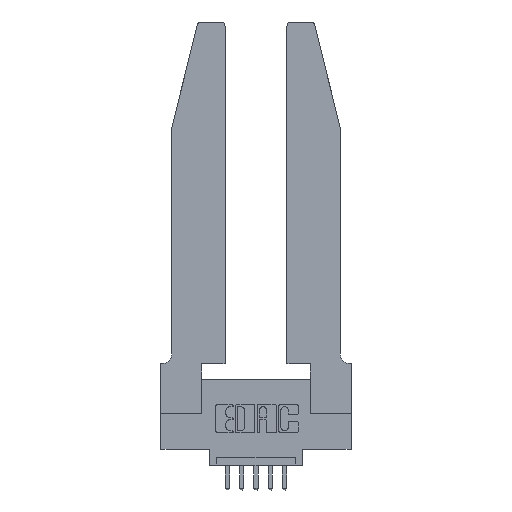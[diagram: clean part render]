
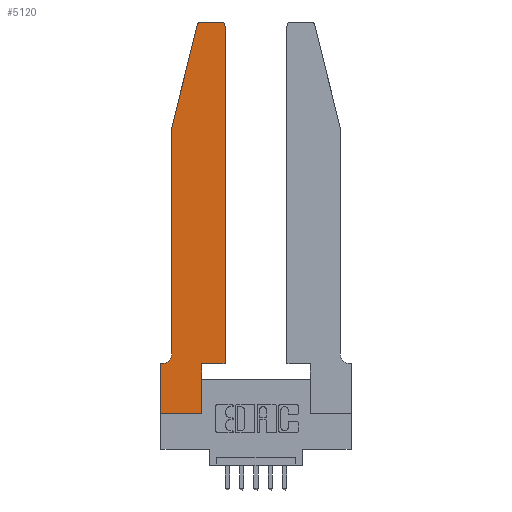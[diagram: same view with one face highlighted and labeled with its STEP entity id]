
A CAD part, top view. The second image highlights one B-rep face of the part: STEP entity #5120.
In plain terms, the highlighted planar face has unit normal (0, 0, 1).
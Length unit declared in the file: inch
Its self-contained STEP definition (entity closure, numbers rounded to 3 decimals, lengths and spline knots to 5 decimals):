
#162 = CARTESIAN_POINT ( 'NONE',  ( 0.2865, 0.35, 0.37 ) ) ;
#192 = EDGE_LOOP ( 'NONE', ( #10039, #7014, #6749, #9158, #2824, #9140, #12492, #2630, #3461, #7036, #6028, #13361 ) ) ;
#282 = CARTESIAN_POINT ( 'NONE',  ( 0., 0.35, 0.37 ) ) ;
#284 = DIRECTION ( 'NONE',  ( -0.239, -0.971, 0. ) ) ;
#394 = VERTEX_POINT ( 'NONE', #13601 ) ;
#401 = LINE ( 'NONE', #1565, #3555 ) ;
#539 = VECTOR ( 'NONE', #2109, 39.37008 ) ;
#833 = VERTEX_POINT ( 'NONE', #4978 ) ;
#885 = DIRECTION ( 'NONE',  ( 0., 0., 1. ) ) ;
#1018 = VECTOR ( 'NONE', #3364, 39.37008 ) ;
#1090 = AXIS2_PLACEMENT_3D ( 'NONE', #282, #4609, #3397 ) ;
#1137 = VERTEX_POINT ( 'NONE', #2534 ) ;
#1203 = VERTEX_POINT ( 'NONE', #13426 ) ;
#1565 = CARTESIAN_POINT ( 'NONE',  ( 0.0755, 0.35, 0.37 ) ) ;
#1767 = VECTOR ( 'NONE', #12735, 39.37008 ) ;
#1770 = VECTOR ( 'NONE', #7680, 39.37008 ) ;
#1950 = AXIS2_PLACEMENT_3D ( 'NONE', #2578, #2714, #5833 ) ;
#2034 = DIRECTION ( 'NONE',  ( 1., 0., 0. ) ) ;
#2109 = DIRECTION ( 'NONE',  ( 0., -1., 0. ) ) ;
#2235 = CARTESIAN_POINT ( 'NONE',  ( 0.2605, 2.75, 0.37 ) ) ;
#2374 = DIRECTION ( 'NONE',  ( -1., 0., 0. ) ) ;
#2534 = CARTESIAN_POINT ( 'NONE',  ( 0.2865, 0.35, 0.37 ) ) ;
#2578 = CARTESIAN_POINT ( 'NONE',  ( 0.4205, 2.72, 0.37 ) ) ;
#2630 = ORIENTED_EDGE ( 'NONE', *, *, #3202, .T. ) ;
#2714 = DIRECTION ( 'NONE',  ( 0., 0., 1. ) ) ;
#2824 = ORIENTED_EDGE ( 'NONE', *, *, #10400, .T. ) ;
#2969 = CARTESIAN_POINT ( 'NONE',  ( 0., 0., 0.37 ) ) ;
#3109 = CARTESIAN_POINT ( 'NONE',  ( 0.284, 2.72, 0.37 ) ) ;
#3128 = LINE ( 'NONE', #13609, #9142 ) ;
#3202 = EDGE_CURVE ( 'NONE', #12722, #394, #4617, .T. ) ;
#3364 = DIRECTION ( 'NONE',  ( 0., 1., 0. ) ) ;
#3397 = DIRECTION ( 'NONE',  ( 1., 0., 0. ) ) ;
#3461 = ORIENTED_EDGE ( 'NONE', *, *, #12194, .T. ) ;
#3555 = VECTOR ( 'NONE', #13127, 39.37008 ) ;
#3591 = VERTEX_POINT ( 'NONE', #9703 ) ;
#3933 = LINE ( 'NONE', #9769, #1770 ) ;
#4102 = DIRECTION ( 'NONE',  ( 1., 0., 0. ) ) ;
#4292 = DIRECTION ( 'NONE',  ( 0., 0., -1. ) ) ;
#4609 = DIRECTION ( 'NONE',  ( 0., 0., 1. ) ) ;
#4617 = LINE ( 'NONE', #2969, #1767 ) ;
#4635 = CARTESIAN_POINT ( 'NONE',  ( 0.0055, 0.35, 0.37 ) ) ;
#4761 = CARTESIAN_POINT ( 'NONE',  ( 0.4205, 2.75, 0.37 ) ) ;
#4847 = VECTOR ( 'NONE', #7416, 39.37008 ) ;
#4978 = CARTESIAN_POINT ( 'NONE',  ( 0.4505, 2.72, 0.37 ) ) ;
#5034 = CARTESIAN_POINT ( 'NONE',  ( 0.284, 2.75, 0.37 ) ) ;
#5111 = CARTESIAN_POINT ( 'NONE',  ( 0., 0., 0.37 ) ) ;
#5120 = ADVANCED_FACE ( 'NONE', ( #7753 ), #7647, .T. ) ;
#5221 = EDGE_CURVE ( 'NONE', #11768, #3591, #401, .T. ) ;
#5291 = CARTESIAN_POINT ( 'NONE',  ( 0., 0., 0.37 ) ) ;
#5505 = CARTESIAN_POINT ( 'NONE',  ( 0.0055, 0.42, 0.37 ) ) ;
#5615 = VECTOR ( 'NONE', #284, 39.37008 ) ;
#5833 = DIRECTION ( 'NONE',  ( 1., 0., 0. ) ) ;
#5857 = EDGE_CURVE ( 'NONE', #833, #11888, #7836, .T. ) ;
#6018 = LINE ( 'NONE', #6808, #13307 ) ;
#6028 = ORIENTED_EDGE ( 'NONE', *, *, #8712, .T. ) ;
#6052 = VERTEX_POINT ( 'NONE', #6056 ) ;
#6056 = CARTESIAN_POINT ( 'NONE',  ( 0.4505, 0.35, 0.37 ) ) ;
#6341 = LINE ( 'NONE', #162, #1018 ) ;
#6537 = LINE ( 'NONE', #5291, #539 ) ;
#6749 = ORIENTED_EDGE ( 'NONE', *, *, #8317, .T. ) ;
#6806 = LINE ( 'NONE', #8716, #5615 ) ;
#6808 = CARTESIAN_POINT ( 'NONE',  ( 0.0755, 2., 0.37 ) ) ;
#7014 = ORIENTED_EDGE ( 'NONE', *, *, #8008, .T. ) ;
#7036 = ORIENTED_EDGE ( 'NONE', *, *, #7482, .T. ) ;
#7416 = DIRECTION ( 'NONE',  ( -1., 0., 0. ) ) ;
#7482 = EDGE_CURVE ( 'NONE', #1137, #6052, #3128, .T. ) ;
#7647 = PLANE ( 'NONE',  #1090 ) ;
#7680 = DIRECTION ( 'NONE',  ( 0., 1., 0. ) ) ;
#7753 = FACE_OUTER_BOUND ( 'NONE', #192, .T. ) ;
#7836 = CIRCLE ( 'NONE', #1950, 0.03 ) ;
#8008 = EDGE_CURVE ( 'NONE', #10188, #1203, #8807, .T. ) ;
#8317 = EDGE_CURVE ( 'NONE', #1203, #11337, #6806, .T. ) ;
#8712 = EDGE_CURVE ( 'NONE', #6052, #833, #3933, .T. ) ;
#8716 = CARTESIAN_POINT ( 'NONE',  ( 0.0755, 2., 0.37 ) ) ;
#8807 = CIRCLE ( 'NONE', #9668, 0.03 ) ;
#9140 = ORIENTED_EDGE ( 'NONE', *, *, #5221, .T. ) ;
#9142 = VECTOR ( 'NONE', #4102, 39.37008 ) ;
#9158 = ORIENTED_EDGE ( 'NONE', *, *, #12592, .T. ) ;
#9229 = CIRCLE ( 'NONE', #11287, 0.07 ) ;
#9329 = LINE ( 'NONE', #2235, #4847 ) ;
#9668 = AXIS2_PLACEMENT_3D ( 'NONE', #3109, #885, #2034 ) ;
#9703 = CARTESIAN_POINT ( 'NONE',  ( 0., 0.35, 0.37 ) ) ;
#9769 = CARTESIAN_POINT ( 'NONE',  ( 0.4505, 0.35, 0.37 ) ) ;
#10039 = ORIENTED_EDGE ( 'NONE', *, *, #12446, .T. ) ;
#10187 = CARTESIAN_POINT ( 'NONE',  ( 0.0755, 2., 0.37 ) ) ;
#10188 = VERTEX_POINT ( 'NONE', #5034 ) ;
#10400 = EDGE_CURVE ( 'NONE', #11312, #11768, #9229, .T. ) ;
#11028 = DIRECTION ( 'NONE',  ( 0., -1., 0. ) ) ;
#11287 = AXIS2_PLACEMENT_3D ( 'NONE', #5505, #4292, #2374 ) ;
#11290 = CARTESIAN_POINT ( 'NONE',  ( 0.0755, 0.42, 0.37 ) ) ;
#11312 = VERTEX_POINT ( 'NONE', #11290 ) ;
#11337 = VERTEX_POINT ( 'NONE', #10187 ) ;
#11533 = EDGE_CURVE ( 'NONE', #3591, #12722, #6537, .T. ) ;
#11768 = VERTEX_POINT ( 'NONE', #4635 ) ;
#11888 = VERTEX_POINT ( 'NONE', #4761 ) ;
#12194 = EDGE_CURVE ( 'NONE', #394, #1137, #6341, .T. ) ;
#12446 = EDGE_CURVE ( 'NONE', #11888, #10188, #9329, .T. ) ;
#12492 = ORIENTED_EDGE ( 'NONE', *, *, #11533, .T. ) ;
#12592 = EDGE_CURVE ( 'NONE', #11337, #11312, #6018, .T. ) ;
#12722 = VERTEX_POINT ( 'NONE', #5111 ) ;
#12735 = DIRECTION ( 'NONE',  ( 1., 0., 0. ) ) ;
#13127 = DIRECTION ( 'NONE',  ( -1., 0., 0. ) ) ;
#13307 = VECTOR ( 'NONE', #11028, 39.37008 ) ;
#13361 = ORIENTED_EDGE ( 'NONE', *, *, #5857, .T. ) ;
#13426 = CARTESIAN_POINT ( 'NONE',  ( 0.25487, 2.72718, 0.37 ) ) ;
#13601 = CARTESIAN_POINT ( 'NONE',  ( 0.2865, 0., 0.37 ) ) ;
#13609 = CARTESIAN_POINT ( 'NONE',  ( 0.4505, 0.35, 0.37 ) ) ;
